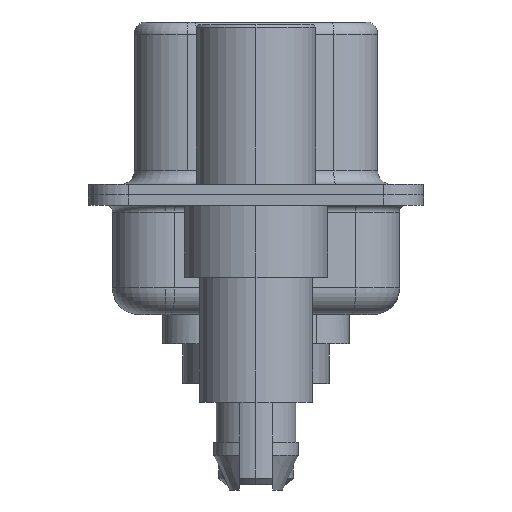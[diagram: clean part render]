
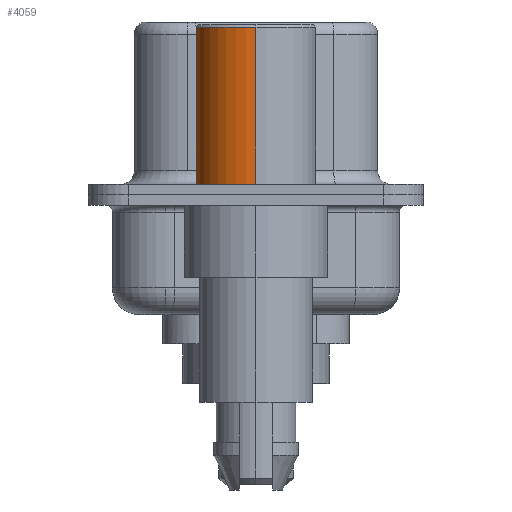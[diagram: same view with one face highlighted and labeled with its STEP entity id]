
A CAD part, left-side view. The second image highlights one B-rep face of the part: STEP entity #4059.
In plain terms, the highlighted cylindrical face has radius 2.25 mm (diameter 4.5 mm), a partial arc.
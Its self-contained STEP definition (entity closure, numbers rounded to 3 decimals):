
#46 = VERTEX_POINT ( 'NONE', #2921 ) ;
#164 = DIRECTION ( 'NONE',  ( 0., 0., 1. ) ) ;
#589 = LINE ( 'NONE', #13226, #4199 ) ;
#766 = EDGE_LOOP ( 'NONE', ( #1000, #17632, #11445, #14169 ) ) ;
#794 = CARTESIAN_POINT ( 'NONE',  ( 0., 0., 0.581 ) ) ;
#1000 = ORIENTED_EDGE ( 'NONE', *, *, #16984, .T. ) ;
#1366 = CIRCLE ( 'NONE', #10660, 2.25 ) ;
#1496 = VERTEX_POINT ( 'NONE', #14574 ) ;
#2802 = CARTESIAN_POINT ( 'NONE',  ( 2.25, 0., 0.4 ) ) ;
#2921 = CARTESIAN_POINT ( 'NONE',  ( -2.25, 0., 6.3 ) ) ;
#3081 = DIRECTION ( 'NONE',  ( 0., 0., 1. ) ) ;
#3977 = VECTOR ( 'NONE', #17863, 1000. ) ;
#4059 = ADVANCED_FACE ( 'NONE', ( #17119 ), #13168, .T. ) ;
#4149 = EDGE_CURVE ( 'NONE', #9015, #17926, #589, .T. ) ;
#4199 = VECTOR ( 'NONE', #11919, 1000. ) ;
#4265 = CARTESIAN_POINT ( 'NONE',  ( 2.25, 0., 6.3 ) ) ;
#4324 = DIRECTION ( 'NONE',  ( 1., 0., 0. ) ) ;
#5289 = CARTESIAN_POINT ( 'NONE',  ( 0., 0., 6.3 ) ) ;
#5580 = CIRCLE ( 'NONE', #6770, 2.25 ) ;
#6757 = DIRECTION ( 'NONE',  ( 1., 0., 0. ) ) ;
#6770 = AXIS2_PLACEMENT_3D ( 'NONE', #5289, #15342, #6757 ) ;
#9015 = VERTEX_POINT ( 'NONE', #2802 ) ;
#9221 = CARTESIAN_POINT ( 'NONE',  ( -2.25, 0., 0.581 ) ) ;
#10660 = AXIS2_PLACEMENT_3D ( 'NONE', #11760, #3081, #13126 ) ;
#10701 = AXIS2_PLACEMENT_3D ( 'NONE', #794, #164, #4324 ) ;
#11445 = ORIENTED_EDGE ( 'NONE', *, *, #15196, .F. ) ;
#11760 = CARTESIAN_POINT ( 'NONE',  ( 0., 0., 0.4 ) ) ;
#11919 = DIRECTION ( 'NONE',  ( 0., 0., 1. ) ) ;
#12127 = LINE ( 'NONE', #9221, #3977 ) ;
#13126 = DIRECTION ( 'NONE',  ( 1., 0., 0. ) ) ;
#13168 = CYLINDRICAL_SURFACE ( 'NONE', #10701, 2.25 ) ;
#13226 = CARTESIAN_POINT ( 'NONE',  ( 2.25, 0., 0.581 ) ) ;
#14169 = ORIENTED_EDGE ( 'NONE', *, *, #4149, .F. ) ;
#14574 = CARTESIAN_POINT ( 'NONE',  ( -2.25, 0., 0.4 ) ) ;
#15196 = EDGE_CURVE ( 'NONE', #17926, #46, #5580, .T. ) ;
#15342 = DIRECTION ( 'NONE',  ( 0., 0., 1. ) ) ;
#16984 = EDGE_CURVE ( 'NONE', #9015, #1496, #1366, .T. ) ;
#17090 = EDGE_CURVE ( 'NONE', #1496, #46, #12127, .T. ) ;
#17119 = FACE_OUTER_BOUND ( 'NONE', #766, .T. ) ;
#17632 = ORIENTED_EDGE ( 'NONE', *, *, #17090, .T. ) ;
#17863 = DIRECTION ( 'NONE',  ( 0., 0., 1. ) ) ;
#17926 = VERTEX_POINT ( 'NONE', #4265 ) ;
